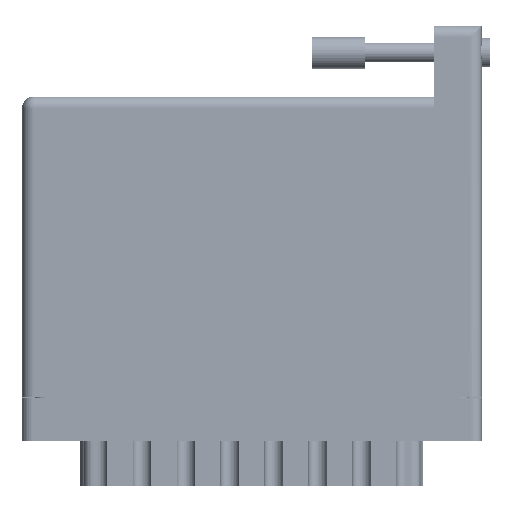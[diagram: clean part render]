
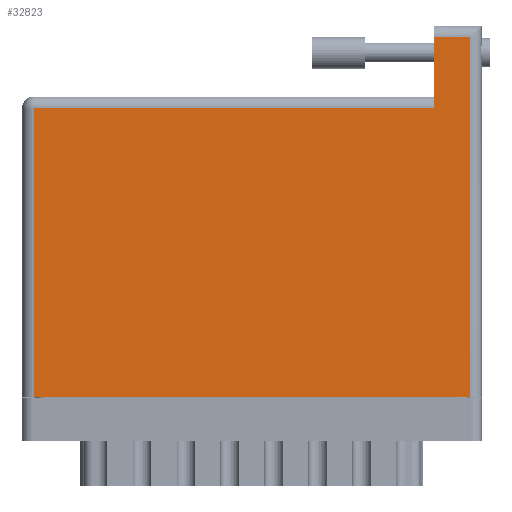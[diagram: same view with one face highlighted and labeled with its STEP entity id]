
A CAD part, front view. The second image highlights one B-rep face of the part: STEP entity #32823.
In plain terms, the highlighted face is planar.
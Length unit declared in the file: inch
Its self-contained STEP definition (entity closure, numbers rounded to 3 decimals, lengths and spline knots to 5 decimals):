
#3017 = DIRECTION ( 'NONE',  ( -1., 0., 0. ) ) ;
#3110 = VECTOR ( 'NONE', #26752, 39.37008 ) ;
#3325 = DIRECTION ( 'NONE',  ( 1., 0., 0. ) ) ;
#3701 = LINE ( 'NONE', #9116, #54860 ) ;
#3992 = CARTESIAN_POINT ( 'NONE',  ( 0.07, 0., 0. ) ) ;
#7717 = CARTESIAN_POINT ( 'NONE',  ( 2.648, 2.195, 0. ) ) ;
#9116 = CARTESIAN_POINT ( 'NONE',  ( 0., 0., 0. ) ) ;
#9340 = AXIS2_PLACEMENT_3D ( 'NONE', #37193, #54962, #14035 ) ;
#9746 = LINE ( 'NONE', #51833, #3110 ) ;
#11156 = ORIENTED_EDGE ( 'NONE', *, *, #42989, .T. ) ;
#11741 = VECTOR ( 'NONE', #28533, 39.37008 ) ;
#13616 = CARTESIAN_POINT ( 'NONE',  ( 2.648, 2.125, 0. ) ) ;
#13666 = FACE_OUTER_BOUND ( 'NONE', #52585, .T. ) ;
#14035 = DIRECTION ( 'NONE',  ( -1., 0., 0. ) ) ;
#14621 = CARTESIAN_POINT ( 'NONE',  ( 0., 1.705, 0. ) ) ;
#17003 = CARTESIAN_POINT ( 'NONE',  ( 0.07, 1.705, 0. ) ) ;
#21622 = CARTESIAN_POINT ( 'NONE',  ( 2.438, 2.125, 0. ) ) ;
#22921 = LINE ( 'NONE', #29092, #39199 ) ;
#24449 = DIRECTION ( 'NONE',  ( 0., -1., 0. ) ) ;
#25016 = EDGE_CURVE ( 'NONE', #48484, #45911, #35929, .T. ) ;
#26752 = DIRECTION ( 'NONE',  ( -1., 0., 0. ) ) ;
#28533 = DIRECTION ( 'NONE',  ( 0., -1., 0. ) ) ;
#29092 = CARTESIAN_POINT ( 'NONE',  ( 2.438, 2.195, 0. ) ) ;
#31690 = EDGE_CURVE ( 'NONE', #43939, #72625, #45559, .T. ) ;
#32823 = ADVANCED_FACE ( 'NONE', ( #13666 ), #60776, .F. ) ;
#33523 = CARTESIAN_POINT ( 'NONE',  ( 2.438, 1.705, 0. ) ) ;
#35929 = LINE ( 'NONE', #7717, #51760 ) ;
#37193 = CARTESIAN_POINT ( 'NONE',  ( 0., 1.775, 0. ) ) ;
#39199 = VECTOR ( 'NONE', #24449, 39.37008 ) ;
#42989 = EDGE_CURVE ( 'NONE', #46636, #43939, #49391, .T. ) ;
#43361 = EDGE_CURVE ( 'NONE', #45911, #72770, #9746, .T. ) ;
#43939 = VERTEX_POINT ( 'NONE', #17003 ) ;
#45559 = LINE ( 'NONE', #64476, #11741 ) ;
#45911 = VERTEX_POINT ( 'NONE', #13616 ) ;
#46636 = VERTEX_POINT ( 'NONE', #33523 ) ;
#47142 = ORIENTED_EDGE ( 'NONE', *, *, #50396, .T. ) ;
#48484 = VERTEX_POINT ( 'NONE', #49257 ) ;
#49257 = CARTESIAN_POINT ( 'NONE',  ( 2.648, 0., 0. ) ) ;
#49391 = LINE ( 'NONE', #14621, #49986 ) ;
#49986 = VECTOR ( 'NONE', #3017, 39.37008 ) ;
#50396 = EDGE_CURVE ( 'NONE', #72625, #48484, #3701, .T. ) ;
#51760 = VECTOR ( 'NONE', #60654, 39.37008 ) ;
#51833 = CARTESIAN_POINT ( 'NONE',  ( 0., 2.125, 0. ) ) ;
#52585 = EDGE_LOOP ( 'NONE', ( #11156, #69220, #47142, #55464, #63643, #69104 ) ) ;
#54860 = VECTOR ( 'NONE', #3325, 39.37008 ) ;
#54962 = DIRECTION ( 'NONE',  ( 0., 0., -1. ) ) ;
#55464 = ORIENTED_EDGE ( 'NONE', *, *, #25016, .T. ) ;
#60654 = DIRECTION ( 'NONE',  ( 0., 1., 0. ) ) ;
#60776 = PLANE ( 'NONE',  #9340 ) ;
#63643 = ORIENTED_EDGE ( 'NONE', *, *, #43361, .T. ) ;
#64476 = CARTESIAN_POINT ( 'NONE',  ( 0.07, 0., 0. ) ) ;
#66852 = EDGE_CURVE ( 'NONE', #72770, #46636, #22921, .T. ) ;
#69104 = ORIENTED_EDGE ( 'NONE', *, *, #66852, .T. ) ;
#69220 = ORIENTED_EDGE ( 'NONE', *, *, #31690, .T. ) ;
#72625 = VERTEX_POINT ( 'NONE', #3992 ) ;
#72770 = VERTEX_POINT ( 'NONE', #21622 ) ;
